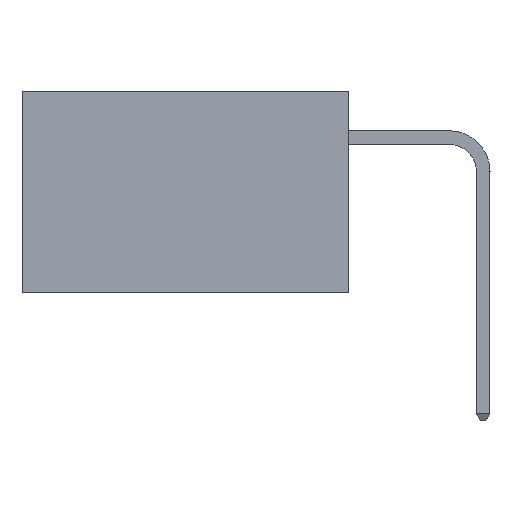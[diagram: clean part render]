
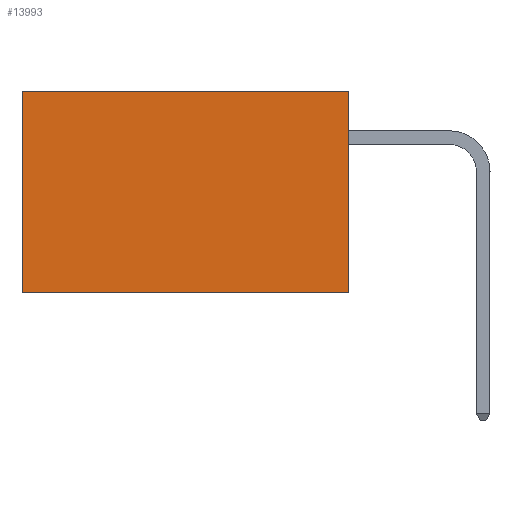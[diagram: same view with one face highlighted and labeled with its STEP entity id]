
A CAD part, left-side view. The second image highlights one B-rep face of the part: STEP entity #13993.
In plain terms, the highlighted planar face has unit normal (-1, 0, 0).
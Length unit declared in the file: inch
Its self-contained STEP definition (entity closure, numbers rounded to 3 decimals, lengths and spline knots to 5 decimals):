
#695 = DIRECTION ( 'NONE',  ( 1., 0., 0. ) ) ;
#2547 = FACE_OUTER_BOUND ( 'NONE', #6294, .T. ) ;
#4870 = CARTESIAN_POINT ( 'NONE',  ( 0.2875, 0.6, 0. ) ) ;
#5831 = ORIENTED_EDGE ( 'NONE', *, *, #13290, .T. ) ;
#6294 = EDGE_LOOP ( 'NONE', ( #33238, #27502, #41028, #5831 ) ) ;
#8309 = PLANE ( 'NONE',  #31342 ) ;
#12153 = CARTESIAN_POINT ( 'NONE',  ( 0.2875, 0., 0. ) ) ;
#13290 = EDGE_CURVE ( 'NONE', #46639, #37284, #30941, .T. ) ;
#13993 = ADVANCED_FACE ( 'NONE', ( #2547 ), #8309, .F. ) ;
#14581 = VECTOR ( 'NONE', #44821, 39.37008 ) ;
#14799 = CARTESIAN_POINT ( 'NONE',  ( 0.2875, 0., -0.37 ) ) ;
#15786 = LINE ( 'NONE', #4870, #20480 ) ;
#16682 = CARTESIAN_POINT ( 'NONE',  ( 0.2875, 0., 0. ) ) ;
#20480 = VECTOR ( 'NONE', #35457, 39.37008 ) ;
#25238 = VECTOR ( 'NONE', #48474, 39.37008 ) ;
#26968 = EDGE_CURVE ( 'NONE', #37284, #40297, #15786, .T. ) ;
#27502 = ORIENTED_EDGE ( 'NONE', *, *, #44569, .F. ) ;
#27552 = LINE ( 'NONE', #14799, #14581 ) ;
#29302 = CARTESIAN_POINT ( 'NONE',  ( 0.2875, 0.6, -0.37 ) ) ;
#29966 = LINE ( 'NONE', #44702, #25238 ) ;
#30941 = LINE ( 'NONE', #12153, #41430 ) ;
#31342 = AXIS2_PLACEMENT_3D ( 'NONE', #34611, #695, #45721 ) ;
#33238 = ORIENTED_EDGE ( 'NONE', *, *, #26968, .T. ) ;
#34611 = CARTESIAN_POINT ( 'NONE',  ( 0.2875, 0., 0. ) ) ;
#35457 = DIRECTION ( 'NONE',  ( 0., 0., -1. ) ) ;
#36037 = VERTEX_POINT ( 'NONE', #45636 ) ;
#37284 = VERTEX_POINT ( 'NONE', #40724 ) ;
#40297 = VERTEX_POINT ( 'NONE', #29302 ) ;
#40724 = CARTESIAN_POINT ( 'NONE',  ( 0.2875, 0.6, 0. ) ) ;
#41028 = ORIENTED_EDGE ( 'NONE', *, *, #43980, .F. ) ;
#41430 = VECTOR ( 'NONE', #42338, 39.37008 ) ;
#42338 = DIRECTION ( 'NONE',  ( 0., 1., 0. ) ) ;
#43980 = EDGE_CURVE ( 'NONE', #46639, #36037, #29966, .T. ) ;
#44569 = EDGE_CURVE ( 'NONE', #36037, #40297, #27552, .T. ) ;
#44702 = CARTESIAN_POINT ( 'NONE',  ( 0.2875, 0., 0. ) ) ;
#44821 = DIRECTION ( 'NONE',  ( 0., 1., 0. ) ) ;
#45636 = CARTESIAN_POINT ( 'NONE',  ( 0.2875, 0., -0.37 ) ) ;
#45721 = DIRECTION ( 'NONE',  ( 0., 0., -1. ) ) ;
#46639 = VERTEX_POINT ( 'NONE', #16682 ) ;
#48474 = DIRECTION ( 'NONE',  ( 0., 0., -1. ) ) ;
